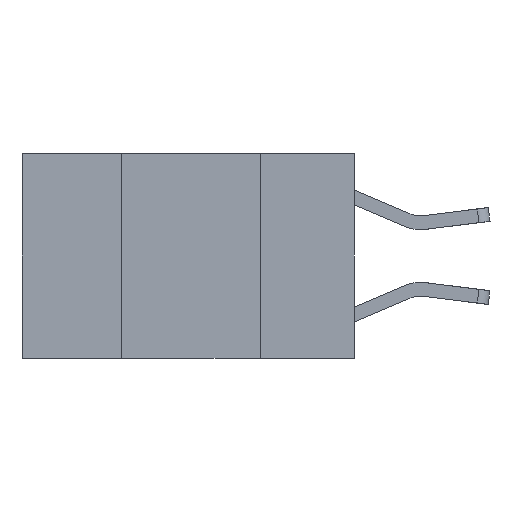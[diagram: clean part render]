
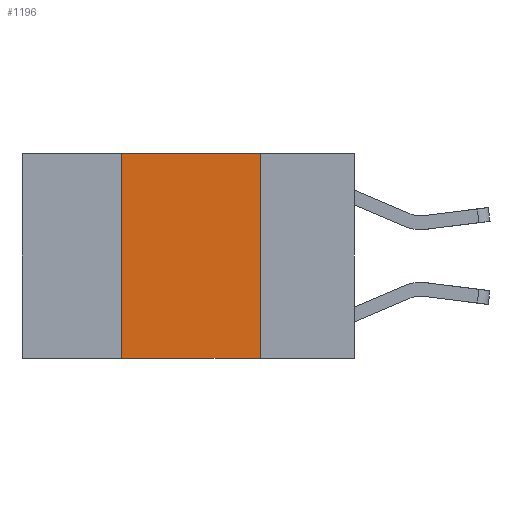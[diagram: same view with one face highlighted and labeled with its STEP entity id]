
A CAD part, left-side view. The second image highlights one B-rep face of the part: STEP entity #1196.
In plain terms, the highlighted planar face has unit normal (-1, 0, 0).
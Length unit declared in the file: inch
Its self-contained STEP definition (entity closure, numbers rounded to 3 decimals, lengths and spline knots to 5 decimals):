
#45 = VECTOR ( 'NONE', #886, 39.37008 ) ;
#177 = CARTESIAN_POINT ( 'NONE',  ( 0., 0.17, 0. ) ) ;
#362 = ORIENTED_EDGE ( 'NONE', *, *, #10135, .F. ) ;
#418 = ORIENTED_EDGE ( 'NONE', *, *, #9987, .F. ) ;
#486 = ORIENTED_EDGE ( 'NONE', *, *, #11609, .F. ) ;
#501 = ORIENTED_EDGE ( 'NONE', *, *, #12640, .T. ) ;
#886 = DIRECTION ( 'NONE',  ( 0., 0., -1. ) ) ;
#992 = VECTOR ( 'NONE', #6148, 39.37008 ) ;
#1196 = ADVANCED_FACE ( 'NONE', ( #7539 ), #9890, .F. ) ;
#1221 = CARTESIAN_POINT ( 'NONE',  ( 0., 0.17, -0.37 ) ) ;
#2010 = DIRECTION ( 'NONE',  ( 0., 0., -1. ) ) ;
#2714 = DIRECTION ( 'NONE',  ( 0., -1., 0. ) ) ;
#3137 = VERTEX_POINT ( 'NONE', #177 ) ;
#4347 = LINE ( 'NONE', #5635, #6348 ) ;
#4824 = LINE ( 'NONE', #11596, #45 ) ;
#5635 = CARTESIAN_POINT ( 'NONE',  ( 0., 0.6, 0. ) ) ;
#5675 = DIRECTION ( 'NONE',  ( 0., -1., 0. ) ) ;
#5994 = CARTESIAN_POINT ( 'NONE',  ( 0., 0.6, 0. ) ) ;
#6148 = DIRECTION ( 'NONE',  ( 0., 0., 1. ) ) ;
#6348 = VECTOR ( 'NONE', #5675, 39.37008 ) ;
#6548 = VERTEX_POINT ( 'NONE', #10130 ) ;
#6800 = CARTESIAN_POINT ( 'NONE',  ( 0., 0.42, 0. ) ) ;
#7539 = FACE_OUTER_BOUND ( 'NONE', #7641, .T. ) ;
#7641 = EDGE_LOOP ( 'NONE', ( #362, #418, #486, #501 ) ) ;
#7670 = LINE ( 'NONE', #11470, #9955 ) ;
#7759 = AXIS2_PLACEMENT_3D ( 'NONE', #5994, #7963, #2010 ) ;
#7963 = DIRECTION ( 'NONE',  ( 1., 0., 0. ) ) ;
#9890 = PLANE ( 'NONE',  #7759 ) ;
#9955 = VECTOR ( 'NONE', #2714, 39.37008 ) ;
#9987 = EDGE_CURVE ( 'NONE', #10836, #3137, #4347, .T. ) ;
#10130 = CARTESIAN_POINT ( 'NONE',  ( 0., 0.42, -0.37 ) ) ;
#10135 = EDGE_CURVE ( 'NONE', #3137, #11093, #4824, .T. ) ;
#10836 = VERTEX_POINT ( 'NONE', #6800 ) ;
#11093 = VERTEX_POINT ( 'NONE', #1221 ) ;
#11152 = LINE ( 'NONE', #11900, #992 ) ;
#11470 = CARTESIAN_POINT ( 'NONE',  ( 0., 0.6, -0.37 ) ) ;
#11596 = CARTESIAN_POINT ( 'NONE',  ( 0., 0.17, 0. ) ) ;
#11609 = EDGE_CURVE ( 'NONE', #6548, #10836, #11152, .T. ) ;
#11900 = CARTESIAN_POINT ( 'NONE',  ( 0., 0.42, 0. ) ) ;
#12640 = EDGE_CURVE ( 'NONE', #6548, #11093, #7670, .T. ) ;
